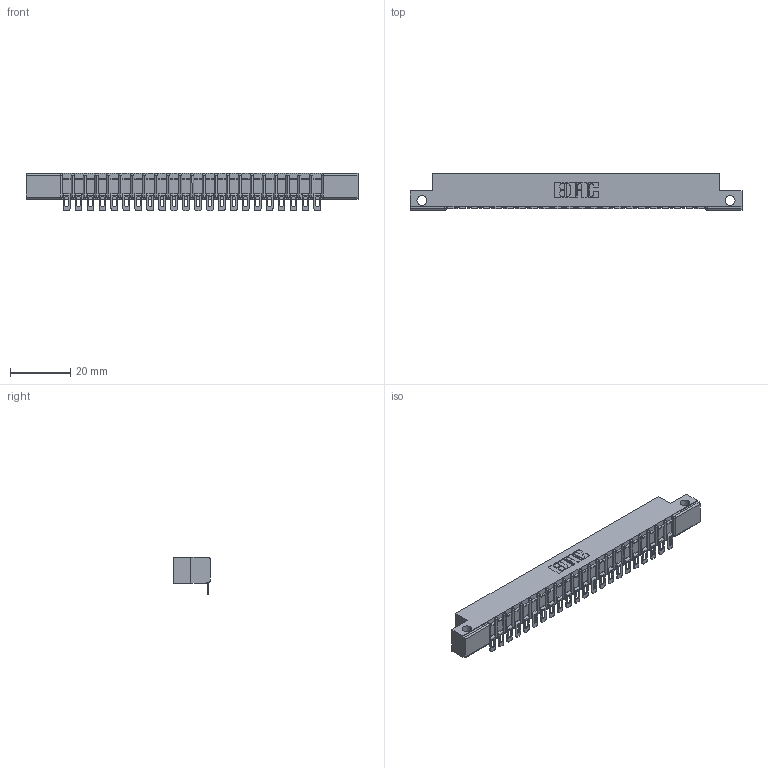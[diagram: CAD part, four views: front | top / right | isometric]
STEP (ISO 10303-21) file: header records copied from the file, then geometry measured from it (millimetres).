
FILE_DESCRIPTION (( 'STEP AP203' ), '1' );
FILE_NAME ('307-022-554-112.STEP', '2018-08-04T03:53:17', ( '' ), ( '' ), 'SwSTEP 2.0', 'SolidWorks 2016', '' );
FILE_SCHEMA (( 'CONFIG_CONTROL_DESIGN' ));
Length unit declared in the file: inch
Products named in the file (3): 307 Part_.128 Dia Side Mounting Holes; 307-290-002_554; 307-022-554-112
Assembly tree (23 placements, depth 2):
  307-022-554-112
    307 Part_.128 Dia Side Mounting Holes
    307-290-002_554  x22
Bounding box: 110.19 x 12.01 x 12.52 mm (x, y, z)
Volume: 7206.2 mm3; surface area: 13059.9 mm2
Topology: 23 solids, 23 shells, 1923 faces, 5889 edges, 3862 vertices
Faces by surface type: plane 1082, cylinder 795, sphere 46
Entity records: 22293 total; most frequent: CARTESIAN_POINT 3758, ORIENTED_EDGE 3748, DIRECTION 3666, EDGE_CURVE 1874, LINE 1418, VECTOR 1418, VERTEX_POINT 1216, AXIS2_PLACEMENT_3D 1124
